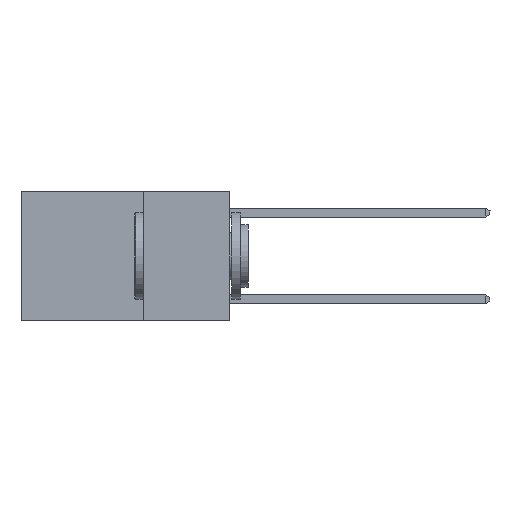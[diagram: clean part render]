
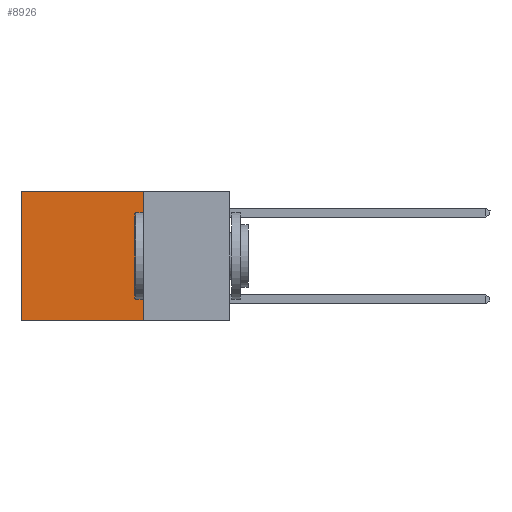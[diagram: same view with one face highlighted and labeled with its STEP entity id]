
A CAD part, left-side view. The second image highlights one B-rep face of the part: STEP entity #8926.
In plain terms, the highlighted planar face has unit normal (-1, 0, 0).
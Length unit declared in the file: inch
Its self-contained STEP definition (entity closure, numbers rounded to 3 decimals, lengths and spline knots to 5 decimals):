
#517 = CARTESIAN_POINT ( 'NONE',  ( 0.2625, 0.25, 0. ) ) ;
#736 = VECTOR ( 'NONE', #17924, 39.37008 ) ;
#1167 = ORIENTED_EDGE ( 'NONE', *, *, #1278, .T. ) ;
#1278 = EDGE_CURVE ( 'NONE', #13564, #1638, #17146, .T. ) ;
#1536 = EDGE_LOOP ( 'NONE', ( #1167, #7591, #2447, #10012 ) ) ;
#1638 = VERTEX_POINT ( 'NONE', #1866 ) ;
#1866 = CARTESIAN_POINT ( 'NONE',  ( 0.2625, 0.6, -0.37 ) ) ;
#1980 = VECTOR ( 'NONE', #16844, 39.37008 ) ;
#2208 = CARTESIAN_POINT ( 'NONE',  ( 0.2625, 0.6, 0. ) ) ;
#2273 = LINE ( 'NONE', #12759, #1980 ) ;
#2447 = ORIENTED_EDGE ( 'NONE', *, *, #5547, .F. ) ;
#3056 = LINE ( 'NONE', #12002, #736 ) ;
#5437 = EDGE_CURVE ( 'NONE', #7701, #1638, #3056, .T. ) ;
#5547 = EDGE_CURVE ( 'NONE', #14067, #7701, #2273, .T. ) ;
#6562 = CARTESIAN_POINT ( 'NONE',  ( 0.2625, 0.6, 0. ) ) ;
#6751 = DIRECTION ( 'NONE',  ( 0., 0., -1. ) ) ;
#7410 = EDGE_CURVE ( 'NONE', #14067, #13564, #14485, .T. ) ;
#7591 = ORIENTED_EDGE ( 'NONE', *, *, #5437, .F. ) ;
#7701 = VERTEX_POINT ( 'NONE', #14082 ) ;
#7885 = AXIS2_PLACEMENT_3D ( 'NONE', #517, #9368, #14122 ) ;
#8926 = ADVANCED_FACE ( 'NONE', ( #18207 ), #14029, .F. ) ;
#9368 = DIRECTION ( 'NONE',  ( 1., 0., 0. ) ) ;
#9478 = CARTESIAN_POINT ( 'NONE',  ( 0.2625, 0.25, 0. ) ) ;
#10012 = ORIENTED_EDGE ( 'NONE', *, *, #7410, .T. ) ;
#10770 = VECTOR ( 'NONE', #14390, 39.37008 ) ;
#12002 = CARTESIAN_POINT ( 'NONE',  ( 0.2625, 0.25, -0.37 ) ) ;
#12759 = CARTESIAN_POINT ( 'NONE',  ( 0.2625, 0.25, 0. ) ) ;
#12837 = CARTESIAN_POINT ( 'NONE',  ( 0.2625, 0.25, 0. ) ) ;
#13564 = VERTEX_POINT ( 'NONE', #2208 ) ;
#14029 = PLANE ( 'NONE',  #7885 ) ;
#14067 = VERTEX_POINT ( 'NONE', #9478 ) ;
#14082 = CARTESIAN_POINT ( 'NONE',  ( 0.2625, 0.25, -0.37 ) ) ;
#14122 = DIRECTION ( 'NONE',  ( 0., 0., -1. ) ) ;
#14390 = DIRECTION ( 'NONE',  ( 0., 1., 0. ) ) ;
#14420 = VECTOR ( 'NONE', #6751, 39.37008 ) ;
#14485 = LINE ( 'NONE', #12837, #10770 ) ;
#16844 = DIRECTION ( 'NONE',  ( 0., 0., -1. ) ) ;
#17146 = LINE ( 'NONE', #6562, #14420 ) ;
#17924 = DIRECTION ( 'NONE',  ( 0., 1., 0. ) ) ;
#18207 = FACE_OUTER_BOUND ( 'NONE', #1536, .T. ) ;
